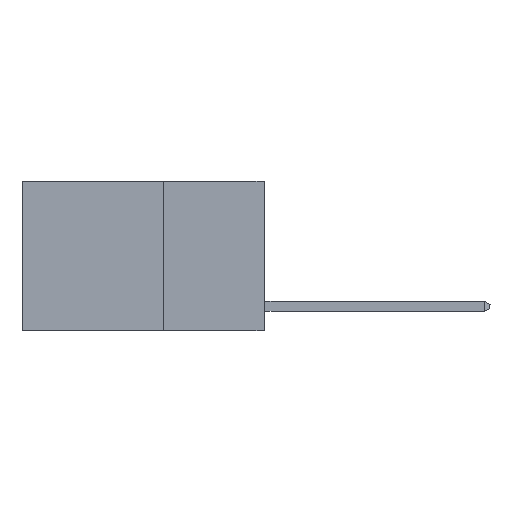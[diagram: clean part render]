
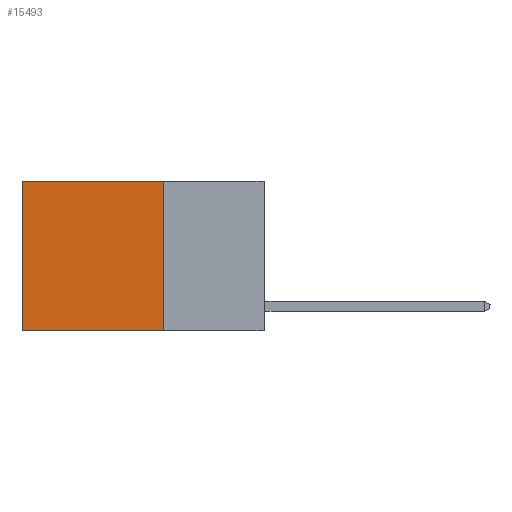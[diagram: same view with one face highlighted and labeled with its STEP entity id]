
A CAD part, left-side view. The second image highlights one B-rep face of the part: STEP entity #15493.
In plain terms, the highlighted planar face has unit normal (-1, 0, 0).
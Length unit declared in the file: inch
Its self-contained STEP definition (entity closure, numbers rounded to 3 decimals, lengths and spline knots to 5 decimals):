
#294 = AXIS2_PLACEMENT_3D ( 'NONE', #12965, #1643, #303 ) ;
#303 = DIRECTION ( 'NONE',  ( 0., 0., -1. ) ) ;
#1041 = DIRECTION ( 'NONE',  ( 0., 1., 0. ) ) ;
#1363 = CARTESIAN_POINT ( 'NONE',  ( 0.2625, 0.25, -0.37 ) ) ;
#1643 = DIRECTION ( 'NONE',  ( 1., 0., 0. ) ) ;
#1664 = LINE ( 'NONE', #15306, #4151 ) ;
#2018 = CARTESIAN_POINT ( 'NONE',  ( 0.2625, 0.6, 0. ) ) ;
#2492 = VERTEX_POINT ( 'NONE', #5222 ) ;
#3975 = CARTESIAN_POINT ( 'NONE',  ( 0.2625, 0.6, -0.37 ) ) ;
#4151 = VECTOR ( 'NONE', #1041, 39.37008 ) ;
#4972 = ORIENTED_EDGE ( 'NONE', *, *, #9923, .T. ) ;
#5222 = CARTESIAN_POINT ( 'NONE',  ( 0.2625, 0.25, 0. ) ) ;
#5305 = EDGE_LOOP ( 'NONE', ( #4972, #12899, #8459, #13080 ) ) ;
#6698 = VECTOR ( 'NONE', #11734, 39.37008 ) ;
#6914 = VECTOR ( 'NONE', #7057, 39.37008 ) ;
#7042 = VERTEX_POINT ( 'NONE', #3975 ) ;
#7057 = DIRECTION ( 'NONE',  ( 0., 1., 0. ) ) ;
#7372 = CARTESIAN_POINT ( 'NONE',  ( 0.2625, 0.25, 0. ) ) ;
#8459 = ORIENTED_EDGE ( 'NONE', *, *, #16177, .F. ) ;
#8633 = VERTEX_POINT ( 'NONE', #15354 ) ;
#9756 = VECTOR ( 'NONE', #13295, 39.37008 ) ;
#9923 = EDGE_CURVE ( 'NONE', #17577, #7042, #17798, .T. ) ;
#10872 = EDGE_CURVE ( 'NONE', #2492, #17577, #1664, .T. ) ;
#11389 = LINE ( 'NONE', #7372, #6698 ) ;
#11575 = PLANE ( 'NONE',  #294 ) ;
#11734 = DIRECTION ( 'NONE',  ( 0., 0., -1. ) ) ;
#11853 = CARTESIAN_POINT ( 'NONE',  ( 0.2625, 0.6, 0. ) ) ;
#12899 = ORIENTED_EDGE ( 'NONE', *, *, #17212, .F. ) ;
#12965 = CARTESIAN_POINT ( 'NONE',  ( 0.2625, 0.25, 0. ) ) ;
#13080 = ORIENTED_EDGE ( 'NONE', *, *, #10872, .T. ) ;
#13295 = DIRECTION ( 'NONE',  ( 0., 0., -1. ) ) ;
#13922 = FACE_OUTER_BOUND ( 'NONE', #5305, .T. ) ;
#15306 = CARTESIAN_POINT ( 'NONE',  ( 0.2625, 0.25, 0. ) ) ;
#15354 = CARTESIAN_POINT ( 'NONE',  ( 0.2625, 0.25, -0.37 ) ) ;
#15493 = ADVANCED_FACE ( 'NONE', ( #13922 ), #11575, .F. ) ;
#16177 = EDGE_CURVE ( 'NONE', #2492, #8633, #11389, .T. ) ;
#16286 = LINE ( 'NONE', #1363, #6914 ) ;
#17212 = EDGE_CURVE ( 'NONE', #8633, #7042, #16286, .T. ) ;
#17577 = VERTEX_POINT ( 'NONE', #11853 ) ;
#17798 = LINE ( 'NONE', #2018, #9756 ) ;
